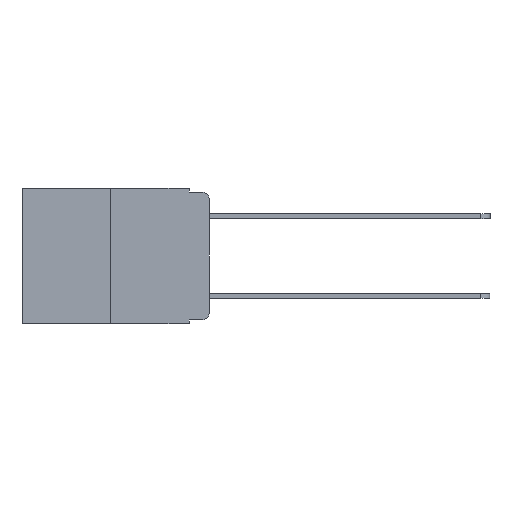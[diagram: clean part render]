
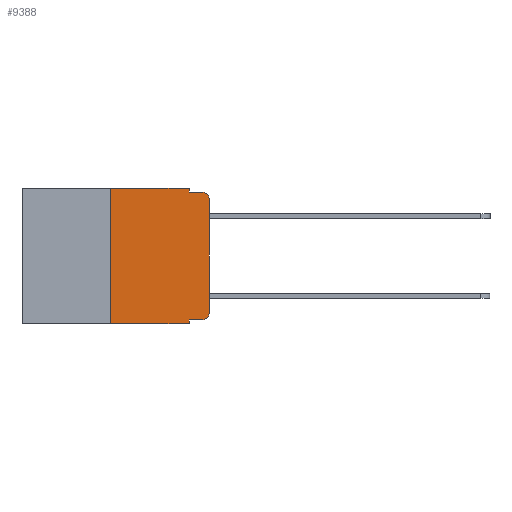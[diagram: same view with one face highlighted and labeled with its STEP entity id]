
A CAD part, left-side view. The second image highlights one B-rep face of the part: STEP entity #9388.
In plain terms, the highlighted planar face has unit normal (-1, 0, 0).
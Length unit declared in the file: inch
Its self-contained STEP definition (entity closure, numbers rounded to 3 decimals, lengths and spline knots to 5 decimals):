
#131 = LINE ( 'NONE', #3997, #6389 ) ;
#193 = DIRECTION ( 'NONE',  ( 0., 0., 1. ) ) ;
#210 = CARTESIAN_POINT ( 'NONE',  ( 0., 0.051, -0.343 ) ) ;
#274 = EDGE_CURVE ( 'NONE', #6339, #406, #873, .T. ) ;
#287 = CARTESIAN_POINT ( 'NONE',  ( 0., 0.051, 0. ) ) ;
#384 = CARTESIAN_POINT ( 'NONE',  ( 0., 0.02, -0.333 ) ) ;
#406 = VERTEX_POINT ( 'NONE', #3932 ) ;
#432 = EDGE_CURVE ( 'NONE', #8746, #3823, #5775, .T. ) ;
#537 = AXIS2_PLACEMENT_3D ( 'NONE', #5626, #6459, #1422 ) ;
#600 = VECTOR ( 'NONE', #6725, 39.37008 ) ;
#618 = AXIS2_PLACEMENT_3D ( 'NONE', #10547, #5881, #798 ) ;
#798 = DIRECTION ( 'NONE',  ( 0., 0., -1. ) ) ;
#828 = CARTESIAN_POINT ( 'NONE',  ( 0., 0.051, 0. ) ) ;
#848 = LINE ( 'NONE', #1552, #5121 ) ;
#873 = LINE ( 'NONE', #7677, #600 ) ;
#958 = VERTEX_POINT ( 'NONE', #6160 ) ;
#1282 = ORIENTED_EDGE ( 'NONE', *, *, #5029, .F. ) ;
#1422 = DIRECTION ( 'NONE',  ( 0., 0., -1. ) ) ;
#1552 = CARTESIAN_POINT ( 'NONE',  ( 0., 0.051, -0.333 ) ) ;
#1872 = CARTESIAN_POINT ( 'NONE',  ( 0., 0.25, 0. ) ) ;
#2099 = CARTESIAN_POINT ( 'NONE',  ( 0., 0.25, 0. ) ) ;
#2137 = CIRCLE ( 'NONE', #3106, 0.02 ) ;
#2284 = VECTOR ( 'NONE', #4182, 39.37008 ) ;
#2405 = ORIENTED_EDGE ( 'NONE', *, *, #8233, .F. ) ;
#2418 = DIRECTION ( 'NONE',  ( 0., -1., 0. ) ) ;
#2738 = VERTEX_POINT ( 'NONE', #6833 ) ;
#2793 = ORIENTED_EDGE ( 'NONE', *, *, #3157, .F. ) ;
#2807 = DIRECTION ( 'NONE',  ( 0., -1., 0. ) ) ;
#2922 = VECTOR ( 'NONE', #2807, 39.37008 ) ;
#3106 = AXIS2_PLACEMENT_3D ( 'NONE', #8682, #3898, #9451 ) ;
#3157 = EDGE_CURVE ( 'NONE', #8887, #9134, #6712, .T. ) ;
#3422 = FACE_OUTER_BOUND ( 'NONE', #4060, .T. ) ;
#3715 = CARTESIAN_POINT ( 'NONE',  ( 0., 0., -0.03 ) ) ;
#3761 = DIRECTION ( 'NONE',  ( 0., 0., -1. ) ) ;
#3823 = VERTEX_POINT ( 'NONE', #3715 ) ;
#3898 = DIRECTION ( 'NONE',  ( -1., 0., 0. ) ) ;
#3932 = CARTESIAN_POINT ( 'NONE',  ( 0., 0.051, 0. ) ) ;
#3943 = EDGE_CURVE ( 'NONE', #3823, #2738, #2137, .T. ) ;
#3952 = VERTEX_POINT ( 'NONE', #384 ) ;
#3997 = CARTESIAN_POINT ( 'NONE',  ( 0., 0.473, -0.343 ) ) ;
#4053 = ORIENTED_EDGE ( 'NONE', *, *, #8566, .T. ) ;
#4060 = EDGE_LOOP ( 'NONE', ( #6502, #5761, #1282, #2405, #5979, #9914, #8894, #2793, #4053, #5717 ) ) ;
#4182 = DIRECTION ( 'NONE',  ( 0., 0., -1. ) ) ;
#4514 = CARTESIAN_POINT ( 'NONE',  ( 0., 0., 0. ) ) ;
#4665 = VERTEX_POINT ( 'NONE', #8739 ) ;
#4807 = PLANE ( 'NONE',  #537 ) ;
#4810 = DIRECTION ( 'NONE',  ( 0., -1., 0. ) ) ;
#5029 = EDGE_CURVE ( 'NONE', #4665, #2738, #5144, .T. ) ;
#5069 = CIRCLE ( 'NONE', #618, 0.02 ) ;
#5121 = VECTOR ( 'NONE', #2418, 39.37008 ) ;
#5144 = LINE ( 'NONE', #8457, #2922 ) ;
#5626 = CARTESIAN_POINT ( 'NONE',  ( 0., 0.473, 0. ) ) ;
#5717 = ORIENTED_EDGE ( 'NONE', *, *, #10612, .T. ) ;
#5761 = ORIENTED_EDGE ( 'NONE', *, *, #3943, .T. ) ;
#5775 = LINE ( 'NONE', #4514, #9467 ) ;
#5881 = DIRECTION ( 'NONE',  ( -1., 0., 0. ) ) ;
#5979 = ORIENTED_EDGE ( 'NONE', *, *, #274, .F. ) ;
#6160 = CARTESIAN_POINT ( 'NONE',  ( 0., 0.25, -0.343 ) ) ;
#6339 = VERTEX_POINT ( 'NONE', #1872 ) ;
#6378 = VECTOR ( 'NONE', #3761, 39.37008 ) ;
#6389 = VECTOR ( 'NONE', #4810, 39.37008 ) ;
#6393 = VECTOR ( 'NONE', #10178, 39.37008 ) ;
#6459 = DIRECTION ( 'NONE',  ( 1., 0., 0. ) ) ;
#6502 = ORIENTED_EDGE ( 'NONE', *, *, #432, .T. ) ;
#6712 = LINE ( 'NONE', #828, #2284 ) ;
#6725 = DIRECTION ( 'NONE',  ( 0., -1., 0. ) ) ;
#6833 = CARTESIAN_POINT ( 'NONE',  ( 0., 0.02, -0.01 ) ) ;
#7025 = LINE ( 'NONE', #287, #6378 ) ;
#7677 = CARTESIAN_POINT ( 'NONE',  ( 0., 0.473, 0. ) ) ;
#7829 = EDGE_CURVE ( 'NONE', #958, #9134, #131, .T. ) ;
#8233 = EDGE_CURVE ( 'NONE', #406, #4665, #7025, .T. ) ;
#8457 = CARTESIAN_POINT ( 'NONE',  ( 0., 0.051, -0.01 ) ) ;
#8566 = EDGE_CURVE ( 'NONE', #8887, #3952, #848, .T. ) ;
#8622 = CARTESIAN_POINT ( 'NONE',  ( 0., 0.051, -0.333 ) ) ;
#8682 = CARTESIAN_POINT ( 'NONE',  ( 0., 0.02, -0.03 ) ) ;
#8708 = LINE ( 'NONE', #2099, #6393 ) ;
#8739 = CARTESIAN_POINT ( 'NONE',  ( 0., 0.051, -0.01 ) ) ;
#8746 = VERTEX_POINT ( 'NONE', #9138 ) ;
#8887 = VERTEX_POINT ( 'NONE', #8622 ) ;
#8894 = ORIENTED_EDGE ( 'NONE', *, *, #7829, .T. ) ;
#9134 = VERTEX_POINT ( 'NONE', #210 ) ;
#9138 = CARTESIAN_POINT ( 'NONE',  ( 0., 0., -0.313 ) ) ;
#9253 = EDGE_CURVE ( 'NONE', #958, #6339, #8708, .T. ) ;
#9388 = ADVANCED_FACE ( 'NONE', ( #3422 ), #4807, .F. ) ;
#9451 = DIRECTION ( 'NONE',  ( 0., 0., -1. ) ) ;
#9467 = VECTOR ( 'NONE', #193, 39.37008 ) ;
#9914 = ORIENTED_EDGE ( 'NONE', *, *, #9253, .F. ) ;
#10178 = DIRECTION ( 'NONE',  ( 0., 0., 1. ) ) ;
#10547 = CARTESIAN_POINT ( 'NONE',  ( 0., 0.02, -0.313 ) ) ;
#10612 = EDGE_CURVE ( 'NONE', #3952, #8746, #5069, .T. ) ;
